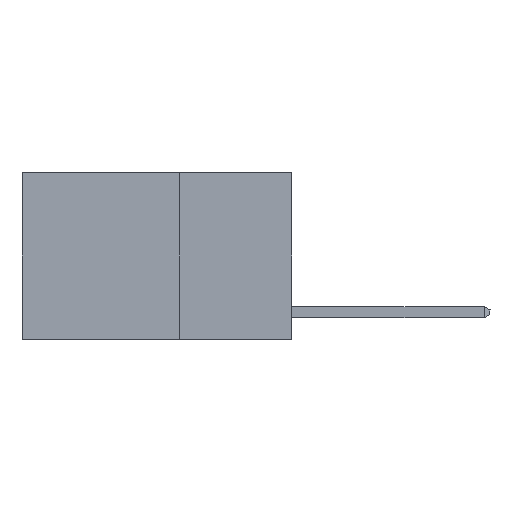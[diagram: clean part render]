
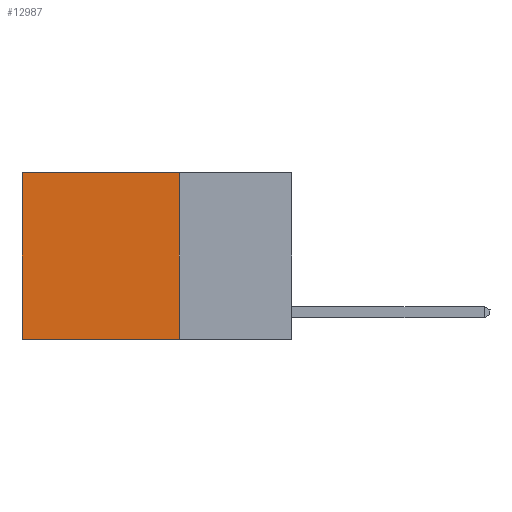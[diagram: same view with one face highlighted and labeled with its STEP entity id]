
A CAD part, left-side view. The second image highlights one B-rep face of the part: STEP entity #12987.
In plain terms, the highlighted planar face has unit normal (-1, 0, 0).
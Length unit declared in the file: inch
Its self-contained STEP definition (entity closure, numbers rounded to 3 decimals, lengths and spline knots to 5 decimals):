
#804 = CARTESIAN_POINT ( 'NONE',  ( 0.2625, 0.6, 0. ) ) ;
#914 = FACE_OUTER_BOUND ( 'NONE', #8891, .T. ) ;
#1882 = VERTEX_POINT ( 'NONE', #9885 ) ;
#2231 = VECTOR ( 'NONE', #16389, 39.37008 ) ;
#2656 = ORIENTED_EDGE ( 'NONE', *, *, #11597, .F. ) ;
#2804 = VERTEX_POINT ( 'NONE', #11721 ) ;
#5374 = EDGE_CURVE ( 'NONE', #13993, #1882, #5659, .T. ) ;
#5659 = LINE ( 'NONE', #14257, #6057 ) ;
#5762 = CARTESIAN_POINT ( 'NONE',  ( 0.2625, 0.25, 0. ) ) ;
#6029 = DIRECTION ( 'NONE',  ( 0., 1., 0. ) ) ;
#6057 = VECTOR ( 'NONE', #13070, 39.37008 ) ;
#6347 = DIRECTION ( 'NONE',  ( 1., 0., 0. ) ) ;
#6942 = LINE ( 'NONE', #804, #8460 ) ;
#8175 = VECTOR ( 'NONE', #6029, 39.37008 ) ;
#8460 = VECTOR ( 'NONE', #10063, 39.37008 ) ;
#8891 = EDGE_LOOP ( 'NONE', ( #14114, #12697, #2656, #9396 ) ) ;
#9200 = CARTESIAN_POINT ( 'NONE',  ( 0.2625, 0.6, -0.37 ) ) ;
#9223 = LINE ( 'NONE', #9787, #2231 ) ;
#9271 = EDGE_CURVE ( 'NONE', #2804, #15218, #14342, .T. ) ;
#9326 = EDGE_CURVE ( 'NONE', #1882, #15218, #6942, .T. ) ;
#9396 = ORIENTED_EDGE ( 'NONE', *, *, #5374, .T. ) ;
#9787 = CARTESIAN_POINT ( 'NONE',  ( 0.2625, 0.25, 0. ) ) ;
#9885 = CARTESIAN_POINT ( 'NONE',  ( 0.2625, 0.6, 0. ) ) ;
#10063 = DIRECTION ( 'NONE',  ( 0., 0., -1. ) ) ;
#11597 = EDGE_CURVE ( 'NONE', #13993, #2804, #9223, .T. ) ;
#11721 = CARTESIAN_POINT ( 'NONE',  ( 0.2625, 0.25, -0.37 ) ) ;
#12697 = ORIENTED_EDGE ( 'NONE', *, *, #9271, .F. ) ;
#12926 = CARTESIAN_POINT ( 'NONE',  ( 0.2625, 0.25, 0. ) ) ;
#12987 = ADVANCED_FACE ( 'NONE', ( #914 ), #14229, .F. ) ;
#13070 = DIRECTION ( 'NONE',  ( 0., 1., 0. ) ) ;
#13906 = CARTESIAN_POINT ( 'NONE',  ( 0.2625, 0.25, -0.37 ) ) ;
#13993 = VERTEX_POINT ( 'NONE', #5762 ) ;
#14114 = ORIENTED_EDGE ( 'NONE', *, *, #9326, .T. ) ;
#14229 = PLANE ( 'NONE',  #15680 ) ;
#14257 = CARTESIAN_POINT ( 'NONE',  ( 0.2625, 0.25, 0. ) ) ;
#14342 = LINE ( 'NONE', #13906, #8175 ) ;
#15218 = VERTEX_POINT ( 'NONE', #9200 ) ;
#15538 = DIRECTION ( 'NONE',  ( 0., 0., -1. ) ) ;
#15680 = AXIS2_PLACEMENT_3D ( 'NONE', #12926, #6347, #15538 ) ;
#16389 = DIRECTION ( 'NONE',  ( 0., 0., -1. ) ) ;
